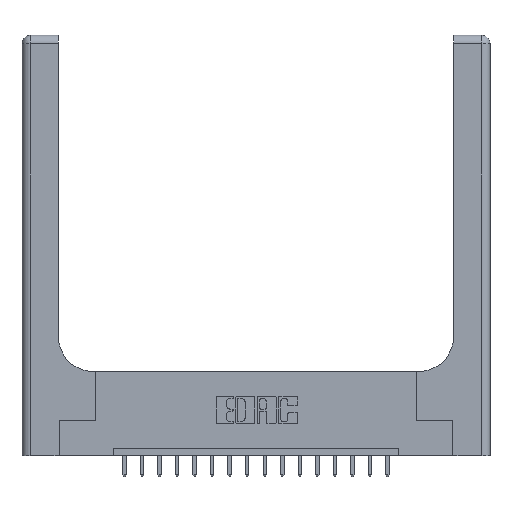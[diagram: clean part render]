
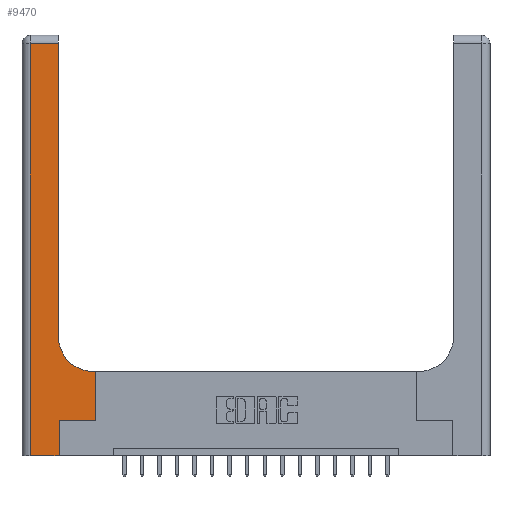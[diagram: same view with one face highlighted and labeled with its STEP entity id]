
A CAD part, top view. The second image highlights one B-rep face of the part: STEP entity #9470.
In plain terms, the highlighted planar face has unit normal (0, 0, 1).
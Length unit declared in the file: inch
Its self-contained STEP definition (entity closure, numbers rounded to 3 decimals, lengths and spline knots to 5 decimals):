
#41 = LINE ( 'NONE', #5923, #4490 ) ;
#134 = DIRECTION ( 'NONE',  ( 0., 1., 0. ) ) ;
#161 = EDGE_CURVE ( 'NONE', #15778, #6068, #16576, .T. ) ;
#518 = CARTESIAN_POINT ( 'NONE',  ( 0.265, 0., 0.37 ) ) ;
#540 = CARTESIAN_POINT ( 'NONE',  ( 0.528, 0.25, 0.37 ) ) ;
#766 = FACE_OUTER_BOUND ( 'NONE', #916, .T. ) ;
#844 = EDGE_CURVE ( 'NONE', #6068, #11838, #5755, .T. ) ;
#916 = EDGE_LOOP ( 'NONE', ( #11909, #4483, #13053, #10025, #2440, #7547, #6135, #9706, #2312 ) ) ;
#1038 = VECTOR ( 'NONE', #134, 39.37008 ) ;
#1513 = EDGE_CURVE ( 'NONE', #10649, #8791, #4979, .T. ) ;
#2137 = VECTOR ( 'NONE', #14972, 39.37008 ) ;
#2312 = ORIENTED_EDGE ( 'NONE', *, *, #161, .T. ) ;
#2440 = ORIENTED_EDGE ( 'NONE', *, *, #12121, .T. ) ;
#2490 = DIRECTION ( 'NONE',  ( 0., 1., 0. ) ) ;
#3194 = CARTESIAN_POINT ( 'NONE',  ( 0.265, 0.25, 0.37 ) ) ;
#3404 = DIRECTION ( 'NONE',  ( 1., 0., 0. ) ) ;
#3533 = DIRECTION ( 'NONE',  ( 1., 0., 0. ) ) ;
#3653 = PLANE ( 'NONE',  #4884 ) ;
#3722 = DIRECTION ( 'NONE',  ( -1., 0., 0. ) ) ;
#3937 = AXIS2_PLACEMENT_3D ( 'NONE', #16526, #15077, #3404 ) ;
#4119 = LINE ( 'NONE', #18681, #9167 ) ;
#4297 = EDGE_CURVE ( 'NONE', #17042, #15778, #16949, .T. ) ;
#4483 = ORIENTED_EDGE ( 'NONE', *, *, #10498, .T. ) ;
#4490 = VECTOR ( 'NONE', #17693, 39.37008 ) ;
#4571 = LINE ( 'NONE', #10425, #18400 ) ;
#4884 = AXIS2_PLACEMENT_3D ( 'NONE', #16582, #9502, #9406 ) ;
#4979 = LINE ( 'NONE', #9383, #16364 ) ;
#5755 = LINE ( 'NONE', #13002, #6472 ) ;
#5816 = EDGE_CURVE ( 'NONE', #6698, #10649, #41, .T. ) ;
#5923 = CARTESIAN_POINT ( 'NONE',  ( 0.06, 3., 0.37 ) ) ;
#6068 = VERTEX_POINT ( 'NONE', #11208 ) ;
#6081 = LINE ( 'NONE', #3194, #2137 ) ;
#6135 = ORIENTED_EDGE ( 'NONE', *, *, #17756, .T. ) ;
#6472 = VECTOR ( 'NONE', #2490, 39.37008 ) ;
#6698 = VERTEX_POINT ( 'NONE', #15998 ) ;
#7547 = ORIENTED_EDGE ( 'NONE', *, *, #16057, .T. ) ;
#7925 = CARTESIAN_POINT ( 'NONE',  ( 0.51, 0.6, 0.37 ) ) ;
#8791 = VERTEX_POINT ( 'NONE', #18160 ) ;
#9167 = VECTOR ( 'NONE', #12633, 39.37008 ) ;
#9383 = CARTESIAN_POINT ( 'NONE',  ( 0., 0., 0.37 ) ) ;
#9406 = DIRECTION ( 'NONE',  ( -1., 0., 0. ) ) ;
#9470 = ADVANCED_FACE ( 'NONE', ( #766 ), #3653, .F. ) ;
#9502 = DIRECTION ( 'NONE',  ( 0., 0., -1. ) ) ;
#9706 = ORIENTED_EDGE ( 'NONE', *, *, #4297, .T. ) ;
#9985 = VERTEX_POINT ( 'NONE', #540 ) ;
#10025 = ORIENTED_EDGE ( 'NONE', *, *, #1513, .T. ) ;
#10063 = CARTESIAN_POINT ( 'NONE',  ( 0.265, 0.25, 0.37 ) ) ;
#10134 = CARTESIAN_POINT ( 'NONE',  ( 0.26, 2.94, 0.37 ) ) ;
#10323 = LINE ( 'NONE', #518, #1038 ) ;
#10425 = CARTESIAN_POINT ( 'NONE',  ( 0., 2.94, 0.37 ) ) ;
#10498 = EDGE_CURVE ( 'NONE', #11838, #6698, #4571, .T. ) ;
#10649 = VERTEX_POINT ( 'NONE', #12394 ) ;
#10848 = CARTESIAN_POINT ( 'NONE',  ( 0.26, 0.6, 0.37 ) ) ;
#11208 = CARTESIAN_POINT ( 'NONE',  ( 0.26, 0.85, 0.37 ) ) ;
#11838 = VERTEX_POINT ( 'NONE', #10134 ) ;
#11909 = ORIENTED_EDGE ( 'NONE', *, *, #844, .T. ) ;
#12121 = EDGE_CURVE ( 'NONE', #8791, #14208, #10323, .T. ) ;
#12394 = CARTESIAN_POINT ( 'NONE',  ( 0.06, 0., 0.37 ) ) ;
#12633 = DIRECTION ( 'NONE',  ( 0., 1., 0. ) ) ;
#13002 = CARTESIAN_POINT ( 'NONE',  ( 0.26, 3., 0.37 ) ) ;
#13053 = ORIENTED_EDGE ( 'NONE', *, *, #5816, .T. ) ;
#14208 = VERTEX_POINT ( 'NONE', #10063 ) ;
#14972 = DIRECTION ( 'NONE',  ( 1., 0., 0. ) ) ;
#14977 = CARTESIAN_POINT ( 'NONE',  ( 0.528, 0.6, 0.37 ) ) ;
#15018 = VECTOR ( 'NONE', #3722, 39.37008 ) ;
#15077 = DIRECTION ( 'NONE',  ( 0., 0., -1. ) ) ;
#15778 = VERTEX_POINT ( 'NONE', #7925 ) ;
#15998 = CARTESIAN_POINT ( 'NONE',  ( 0.06, 2.94, 0.37 ) ) ;
#16057 = EDGE_CURVE ( 'NONE', #14208, #9985, #6081, .T. ) ;
#16348 = DIRECTION ( 'NONE',  ( -1., 0., 0. ) ) ;
#16364 = VECTOR ( 'NONE', #3533, 39.37008 ) ;
#16526 = CARTESIAN_POINT ( 'NONE',  ( 0.51, 0.85, 0.37 ) ) ;
#16576 = CIRCLE ( 'NONE', #3937, 0.25 ) ;
#16582 = CARTESIAN_POINT ( 'NONE',  ( 0., 3., 0.37 ) ) ;
#16949 = LINE ( 'NONE', #10848, #15018 ) ;
#17042 = VERTEX_POINT ( 'NONE', #14977 ) ;
#17693 = DIRECTION ( 'NONE',  ( 0., -1., 0. ) ) ;
#17756 = EDGE_CURVE ( 'NONE', #9985, #17042, #4119, .T. ) ;
#18160 = CARTESIAN_POINT ( 'NONE',  ( 0.265, 0., 0.37 ) ) ;
#18400 = VECTOR ( 'NONE', #16348, 39.37008 ) ;
#18681 = CARTESIAN_POINT ( 'NONE',  ( 0.528, 0.25, 0.37 ) ) ;
